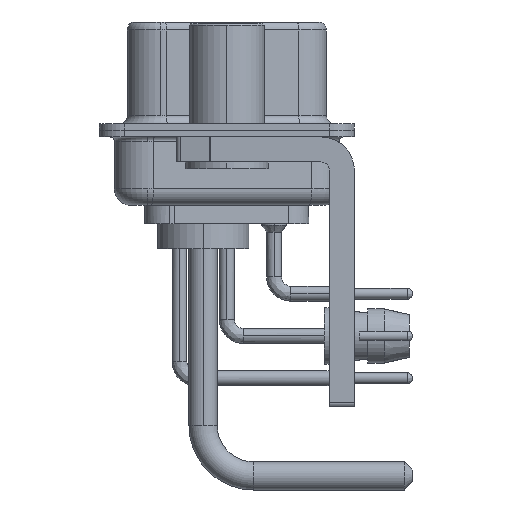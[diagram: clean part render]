
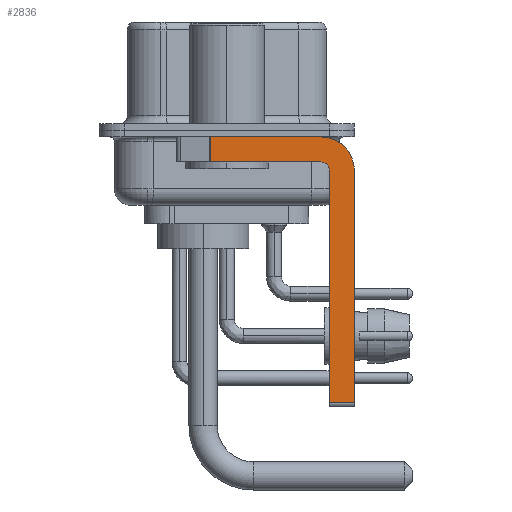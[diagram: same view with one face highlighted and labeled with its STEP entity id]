
A CAD part, left-side view. The second image highlights one B-rep face of the part: STEP entity #2836.
In plain terms, the highlighted planar face has unit normal (-1, 0, 0).
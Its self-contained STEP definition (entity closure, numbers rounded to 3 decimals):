
#794 = ORIENTED_EDGE ( 'NONE', *, *, #7599, .F. ) ;
#1898 = LINE ( 'NONE', #34341, #12183 ) ;
#2240 = DIRECTION ( 'NONE',  ( 0., 0., 1. ) ) ;
#2549 = CARTESIAN_POINT ( 'NONE',  ( -2.9, 0.978, -1.9 ) ) ;
#2634 = DIRECTION ( 'NONE',  ( 1., 0., 0. ) ) ;
#2836 = ADVANCED_FACE ( 'NONE', ( #22343 ), #37251, .F. ) ;
#3125 = ORIENTED_EDGE ( 'NONE', *, *, #34360, .T. ) ;
#3132 = CARTESIAN_POINT ( 'NONE',  ( -2.9, 0.978, -0.4 ) ) ;
#3180 = EDGE_CURVE ( 'NONE', #12726, #20233, #24246, .T. ) ;
#3395 = EDGE_CURVE ( 'NONE', #17784, #15309, #8823, .T. ) ;
#4087 = ORIENTED_EDGE ( 'NONE', *, *, #9651, .T. ) ;
#4829 = CARTESIAN_POINT ( 'NONE',  ( -2.9, -5.65, -2.4 ) ) ;
#6267 = DIRECTION ( 'NONE',  ( 0., 0., 1. ) ) ;
#6851 = CIRCLE ( 'NONE', #28582, 2. ) ;
#6973 = CARTESIAN_POINT ( 'NONE',  ( -2.9, -5.65, -1.9 ) ) ;
#7560 = CARTESIAN_POINT ( 'NONE',  ( -2.9, -6.15, -16.35 ) ) ;
#7599 = EDGE_CURVE ( 'NONE', #9923, #38190, #1898, .T. ) ;
#7949 = DIRECTION ( 'NONE',  ( 1., 0., 0. ) ) ;
#8380 = EDGE_CURVE ( 'NONE', #24909, #17784, #25763, .T. ) ;
#8823 = CIRCLE ( 'NONE', #32363, 0.5 ) ;
#9651 = EDGE_CURVE ( 'NONE', #9923, #29385, #21643, .T. ) ;
#9713 = DIRECTION ( 'NONE',  ( 0., 1., 0. ) ) ;
#9923 = VERTEX_POINT ( 'NONE', #3132 ) ;
#10399 = CARTESIAN_POINT ( 'NONE',  ( -2.9, -5.65, -16.35 ) ) ;
#10560 = EDGE_CURVE ( 'NONE', #15309, #29385, #30863, .T. ) ;
#10587 = LINE ( 'NONE', #10399, #37569 ) ;
#11232 = VECTOR ( 'NONE', #2240, 1000. ) ;
#12084 = CARTESIAN_POINT ( 'NONE',  ( -2.9, -7.65, -2.4 ) ) ;
#12183 = VECTOR ( 'NONE', #37043, 1000. ) ;
#12726 = VERTEX_POINT ( 'NONE', #12084 ) ;
#13749 = VECTOR ( 'NONE', #15797, 1000. ) ;
#14618 = DIRECTION ( 'NONE',  ( -1., 0., 0. ) ) ;
#14875 = EDGE_LOOP ( 'NONE', ( #794, #4087, #29741, #18158, #27803, #3125, #36087, #22670 ) ) ;
#15309 = VERTEX_POINT ( 'NONE', #38346 ) ;
#15797 = DIRECTION ( 'NONE',  ( 0., 0., -1. ) ) ;
#17004 = CARTESIAN_POINT ( 'NONE',  ( -2.9, -6.15, -16.6 ) ) ;
#17784 = VERTEX_POINT ( 'NONE', #30771 ) ;
#17930 = CARTESIAN_POINT ( 'NONE',  ( -2.9, -5.65, -0.4 ) ) ;
#18158 = ORIENTED_EDGE ( 'NONE', *, *, #3395, .F. ) ;
#18728 = CARTESIAN_POINT ( 'NONE',  ( -2.9, 0.978, -1.9 ) ) ;
#20233 = VERTEX_POINT ( 'NONE', #23051 ) ;
#20571 = AXIS2_PLACEMENT_3D ( 'NONE', #4829, #7949, #34543 ) ;
#21643 = LINE ( 'NONE', #18728, #13749 ) ;
#22343 = FACE_OUTER_BOUND ( 'NONE', #14875, .T. ) ;
#22455 = DIRECTION ( 'NONE',  ( 0., -1., 0. ) ) ;
#22670 = ORIENTED_EDGE ( 'NONE', *, *, #27377, .F. ) ;
#23051 = CARTESIAN_POINT ( 'NONE',  ( -2.9, -7.65, -16.35 ) ) ;
#24246 = LINE ( 'NONE', #36064, #34809 ) ;
#24909 = VERTEX_POINT ( 'NONE', #7560 ) ;
#25763 = LINE ( 'NONE', #17004, #11232 ) ;
#27377 = EDGE_CURVE ( 'NONE', #38190, #12726, #6851, .T. ) ;
#27803 = ORIENTED_EDGE ( 'NONE', *, *, #8380, .F. ) ;
#28582 = AXIS2_PLACEMENT_3D ( 'NONE', #37960, #2634, #35442 ) ;
#29385 = VERTEX_POINT ( 'NONE', #2549 ) ;
#29741 = ORIENTED_EDGE ( 'NONE', *, *, #10560, .F. ) ;
#30771 = CARTESIAN_POINT ( 'NONE',  ( -2.9, -6.15, -2.4 ) ) ;
#30863 = LINE ( 'NONE', #6973, #32240 ) ;
#32240 = VECTOR ( 'NONE', #9713, 1000. ) ;
#32363 = AXIS2_PLACEMENT_3D ( 'NONE', #32872, #14618, #6267 ) ;
#32872 = CARTESIAN_POINT ( 'NONE',  ( -2.9, -5.65, -2.4 ) ) ;
#34341 = CARTESIAN_POINT ( 'NONE',  ( -2.9, 3., -0.4 ) ) ;
#34360 = EDGE_CURVE ( 'NONE', #24909, #20233, #10587, .T. ) ;
#34543 = DIRECTION ( 'NONE',  ( 0., 0., -1. ) ) ;
#34809 = VECTOR ( 'NONE', #35871, 1000. ) ;
#35442 = DIRECTION ( 'NONE',  ( 0., 0., -1. ) ) ;
#35871 = DIRECTION ( 'NONE',  ( 0., 0., -1. ) ) ;
#36064 = CARTESIAN_POINT ( 'NONE',  ( -2.9, -7.65, -2.4 ) ) ;
#36087 = ORIENTED_EDGE ( 'NONE', *, *, #3180, .F. ) ;
#37043 = DIRECTION ( 'NONE',  ( 0., -1., 0. ) ) ;
#37251 = PLANE ( 'NONE',  #20571 ) ;
#37569 = VECTOR ( 'NONE', #22455, 1000. ) ;
#37960 = CARTESIAN_POINT ( 'NONE',  ( -2.9, -5.65, -2.4 ) ) ;
#38190 = VERTEX_POINT ( 'NONE', #17930 ) ;
#38346 = CARTESIAN_POINT ( 'NONE',  ( -2.9, -5.65, -1.9 ) ) ;
